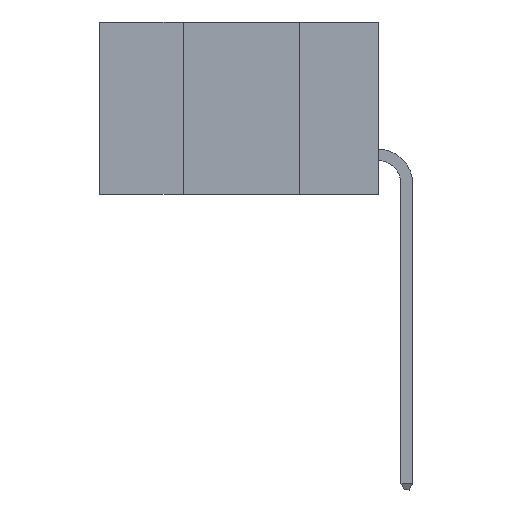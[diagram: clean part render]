
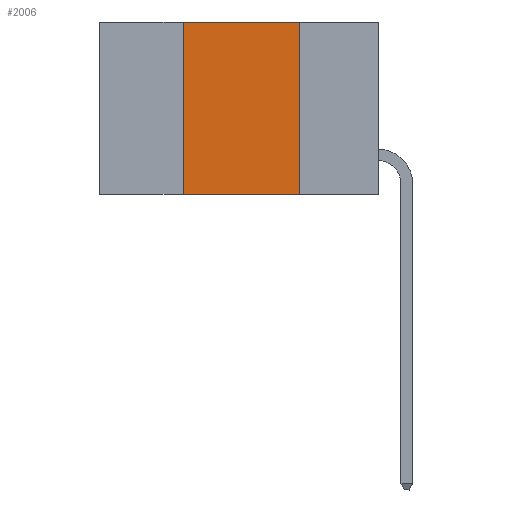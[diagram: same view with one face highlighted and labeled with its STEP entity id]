
A CAD part, left-side view. The second image highlights one B-rep face of the part: STEP entity #2006.
In plain terms, the highlighted planar face has unit normal (-1, 0, 0).
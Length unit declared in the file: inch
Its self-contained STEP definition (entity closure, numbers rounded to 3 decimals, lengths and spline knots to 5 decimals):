
#156 = FACE_OUTER_BOUND ( 'NONE', #10368, .T. ) ;
#1221 = CARTESIAN_POINT ( 'NONE',  ( 0., 0.6, 0. ) ) ;
#2006 = ADVANCED_FACE ( 'NONE', ( #156 ), #6509, .F. ) ;
#2339 = ORIENTED_EDGE ( 'NONE', *, *, #18620, .F. ) ;
#4129 = VECTOR ( 'NONE', #4358, 39.37008 ) ;
#4358 = DIRECTION ( 'NONE',  ( 0., -1., 0. ) ) ;
#4368 = CARTESIAN_POINT ( 'NONE',  ( 0., 0.17, 0. ) ) ;
#6509 = PLANE ( 'NONE',  #7564 ) ;
#7564 = AXIS2_PLACEMENT_3D ( 'NONE', #19762, #21630, #10322 ) ;
#8474 = LINE ( 'NONE', #13535, #17954 ) ;
#9817 = CARTESIAN_POINT ( 'NONE',  ( 0., 0.17, -0.37 ) ) ;
#10322 = DIRECTION ( 'NONE',  ( 0., 0., -1. ) ) ;
#10368 = EDGE_LOOP ( 'NONE', ( #21957, #2339, #13070, #18164 ) ) ;
#10410 = LINE ( 'NONE', #17691, #4129 ) ;
#10477 = LINE ( 'NONE', #16897, #19375 ) ;
#10928 = CARTESIAN_POINT ( 'NONE',  ( 0., 0.42, -0.37 ) ) ;
#11111 = EDGE_CURVE ( 'NONE', #21913, #11819, #10410, .T. ) ;
#11819 = VERTEX_POINT ( 'NONE', #9817 ) ;
#13070 = ORIENTED_EDGE ( 'NONE', *, *, #16232, .F. ) ;
#13423 = VECTOR ( 'NONE', #16493, 39.37008 ) ;
#13535 = CARTESIAN_POINT ( 'NONE',  ( 0., 0.42, 0. ) ) ;
#14107 = VERTEX_POINT ( 'NONE', #4368 ) ;
#15461 = DIRECTION ( 'NONE',  ( 0., 0., 1. ) ) ;
#16232 = EDGE_CURVE ( 'NONE', #21913, #20074, #8474, .T. ) ;
#16493 = DIRECTION ( 'NONE',  ( 0., -1., 0. ) ) ;
#16897 = CARTESIAN_POINT ( 'NONE',  ( 0., 0.17, 0. ) ) ;
#17691 = CARTESIAN_POINT ( 'NONE',  ( 0., 0.6, -0.37 ) ) ;
#17954 = VECTOR ( 'NONE', #15461, 39.37008 ) ;
#18164 = ORIENTED_EDGE ( 'NONE', *, *, #11111, .T. ) ;
#18620 = EDGE_CURVE ( 'NONE', #20074, #14107, #19076, .T. ) ;
#18743 = EDGE_CURVE ( 'NONE', #14107, #11819, #10477, .T. ) ;
#19053 = CARTESIAN_POINT ( 'NONE',  ( 0., 0.42, 0. ) ) ;
#19076 = LINE ( 'NONE', #1221, #13423 ) ;
#19375 = VECTOR ( 'NONE', #24379, 39.37008 ) ;
#19762 = CARTESIAN_POINT ( 'NONE',  ( 0., 0.6, 0. ) ) ;
#20074 = VERTEX_POINT ( 'NONE', #19053 ) ;
#21630 = DIRECTION ( 'NONE',  ( 1., 0., 0. ) ) ;
#21913 = VERTEX_POINT ( 'NONE', #10928 ) ;
#21957 = ORIENTED_EDGE ( 'NONE', *, *, #18743, .F. ) ;
#24379 = DIRECTION ( 'NONE',  ( 0., 0., -1. ) ) ;
